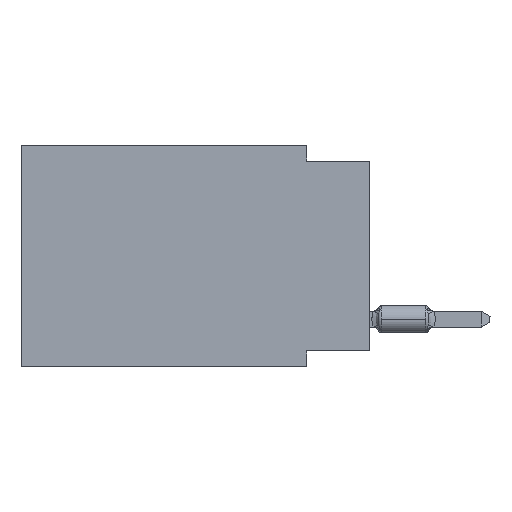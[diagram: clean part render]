
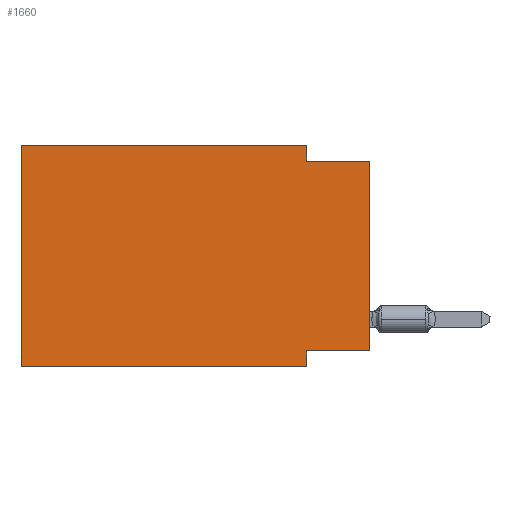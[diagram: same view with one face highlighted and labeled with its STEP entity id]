
A CAD part, left-side view. The second image highlights one B-rep face of the part: STEP entity #1660.
In plain terms, the highlighted planar face has unit normal (-1, 0, 0).
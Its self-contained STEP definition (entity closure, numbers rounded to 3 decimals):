
#1660 = ADVANCED_FACE ( 'NONE', ( #42272 ), #51059, .F. ) ;
#1996 = EDGE_CURVE ( 'NONE', #37619, #47590, #59031, .T. ) ;
#7985 = VECTOR ( 'NONE', #83220, 1000. ) ;
#12830 = VECTOR ( 'NONE', #45405, 1000. ) ;
#14431 = EDGE_CURVE ( 'NONE', #47590, #80309, #85264, .T. ) ;
#14510 = VECTOR ( 'NONE', #59466, 1000. ) ;
#14817 = LINE ( 'NONE', #64282, #94329 ) ;
#17328 = EDGE_CURVE ( 'NONE', #34831, #37619, #105675, .T. ) ;
#19621 = CARTESIAN_POINT ( 'NONE',  ( 0., 2.54, -8.89 ) ) ;
#20879 = VERTEX_POINT ( 'NONE', #31685 ) ;
#24450 = DIRECTION ( 'NONE',  ( 0., 1., 0. ) ) ;
#25219 = CARTESIAN_POINT ( 'NONE',  ( 0., 13.97, 0. ) ) ;
#31685 = CARTESIAN_POINT ( 'NONE',  ( 0., 2.54, -8.89 ) ) ;
#31864 = CARTESIAN_POINT ( 'NONE',  ( 0., 0., -0.635 ) ) ;
#32019 = DIRECTION ( 'NONE',  ( 0., 0., 1. ) ) ;
#32655 = DIRECTION ( 'NONE',  ( 0., -1., 0. ) ) ;
#32671 = CARTESIAN_POINT ( 'NONE',  ( 0., 0., 0. ) ) ;
#32701 = LINE ( 'NONE', #101361, #63386 ) ;
#34831 = VERTEX_POINT ( 'NONE', #61907 ) ;
#37360 = VERTEX_POINT ( 'NONE', #31864 ) ;
#37619 = VERTEX_POINT ( 'NONE', #70800 ) ;
#41912 = VECTOR ( 'NONE', #59773, 1000. ) ;
#42272 = FACE_OUTER_BOUND ( 'NONE', #81282, .T. ) ;
#45405 = DIRECTION ( 'NONE',  ( 0., -1., 0. ) ) ;
#45751 = VECTOR ( 'NONE', #32655, 1000. ) ;
#47590 = VERTEX_POINT ( 'NONE', #105182 ) ;
#48041 = VERTEX_POINT ( 'NONE', #75792 ) ;
#48533 = EDGE_CURVE ( 'NONE', #34831, #20879, #60799, .T. ) ;
#49566 = ORIENTED_EDGE ( 'NONE', *, *, #1996, .F. ) ;
#51059 = PLANE ( 'NONE',  #96541 ) ;
#54000 = ORIENTED_EDGE ( 'NONE', *, *, #59289, .F. ) ;
#54138 = DIRECTION ( 'NONE',  ( 1., 0., 0. ) ) ;
#54586 = CARTESIAN_POINT ( 'NONE',  ( 0., 13.97, 0. ) ) ;
#54979 = EDGE_CURVE ( 'NONE', #48041, #37360, #99169, .T. ) ;
#58185 = ORIENTED_EDGE ( 'NONE', *, *, #48533, .T. ) ;
#58754 = DIRECTION ( 'NONE',  ( 0., 0., -1. ) ) ;
#59031 = LINE ( 'NONE', #83745, #45751 ) ;
#59289 = EDGE_CURVE ( 'NONE', #80309, #37360, #14817, .T. ) ;
#59466 = DIRECTION ( 'NONE',  ( 0., 0., -1. ) ) ;
#59773 = DIRECTION ( 'NONE',  ( 0., 0., -1. ) ) ;
#60799 = LINE ( 'NONE', #94297, #12830 ) ;
#61907 = CARTESIAN_POINT ( 'NONE',  ( 0., 13.97, -8.89 ) ) ;
#63386 = VECTOR ( 'NONE', #24450, 1000. ) ;
#63844 = ORIENTED_EDGE ( 'NONE', *, *, #14431, .F. ) ;
#64282 = CARTESIAN_POINT ( 'NONE',  ( 0., 0., -0.635 ) ) ;
#67169 = CARTESIAN_POINT ( 'NONE',  ( 0., 2.54, 0. ) ) ;
#70800 = CARTESIAN_POINT ( 'NONE',  ( 0., 13.97, 0. ) ) ;
#73347 = ORIENTED_EDGE ( 'NONE', *, *, #17328, .F. ) ;
#75792 = CARTESIAN_POINT ( 'NONE',  ( 0., 0., -8.255 ) ) ;
#76284 = CARTESIAN_POINT ( 'NONE',  ( 0., 2.54, -0.635 ) ) ;
#77327 = LINE ( 'NONE', #19621, #41912 ) ;
#78308 = ORIENTED_EDGE ( 'NONE', *, *, #86898, .F. ) ;
#80309 = VERTEX_POINT ( 'NONE', #76284 ) ;
#81282 = EDGE_LOOP ( 'NONE', ( #108547, #54000, #63844, #49566, #73347, #58185, #78308, #91153 ) ) ;
#83220 = DIRECTION ( 'NONE',  ( 0., 0., 1. ) ) ;
#83745 = CARTESIAN_POINT ( 'NONE',  ( 0., 13.97, 0. ) ) ;
#85264 = LINE ( 'NONE', #67169, #14510 ) ;
#86898 = EDGE_CURVE ( 'NONE', #92411, #20879, #77327, .T. ) ;
#91153 = ORIENTED_EDGE ( 'NONE', *, *, #95079, .F. ) ;
#92411 = VERTEX_POINT ( 'NONE', #101381 ) ;
#94297 = CARTESIAN_POINT ( 'NONE',  ( 0., 13.97, -8.89 ) ) ;
#94329 = VECTOR ( 'NONE', #104953, 1000. ) ;
#95079 = EDGE_CURVE ( 'NONE', #48041, #92411, #32701, .T. ) ;
#96541 = AXIS2_PLACEMENT_3D ( 'NONE', #25219, #54138, #58754 ) ;
#99169 = LINE ( 'NONE', #32671, #7985 ) ;
#101361 = CARTESIAN_POINT ( 'NONE',  ( 0., 0., -8.255 ) ) ;
#101381 = CARTESIAN_POINT ( 'NONE',  ( 0., 2.54, -8.255 ) ) ;
#102752 = VECTOR ( 'NONE', #32019, 1000. ) ;
#104953 = DIRECTION ( 'NONE',  ( 0., -1., 0. ) ) ;
#105182 = CARTESIAN_POINT ( 'NONE',  ( 0., 2.54, 0. ) ) ;
#105675 = LINE ( 'NONE', #54586, #102752 ) ;
#108547 = ORIENTED_EDGE ( 'NONE', *, *, #54979, .T. ) ;
